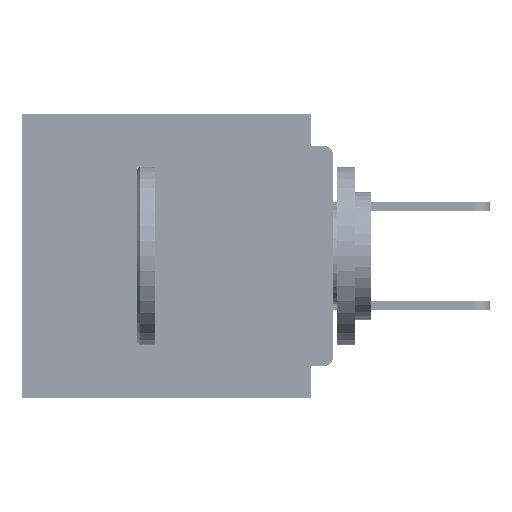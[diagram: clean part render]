
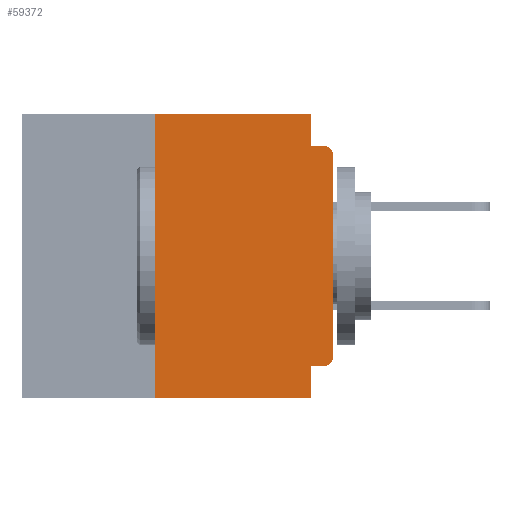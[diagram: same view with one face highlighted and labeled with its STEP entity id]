
A CAD part, left-side view. The second image highlights one B-rep face of the part: STEP entity #59372.
In plain terms, the highlighted planar face has unit normal (-1, 0, 0).
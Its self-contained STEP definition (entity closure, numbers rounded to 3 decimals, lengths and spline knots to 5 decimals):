
#410 = ORIENTED_EDGE ( 'NONE', *, *, #3255, .T. ) ;
#1782 = CARTESIAN_POINT ( 'NONE',  ( 0., 0.437, 0. ) ) ;
#1828 = CARTESIAN_POINT ( 'NONE',  ( 0., 0.437, -0.4 ) ) ;
#3255 = EDGE_CURVE ( 'NONE', #49868, #56918, #58562, .T. ) ;
#4190 = EDGE_CURVE ( 'NONE', #19603, #50509, #42094, .T. ) ;
#5591 = LINE ( 'NONE', #66463, #33182 ) ;
#6256 = DIRECTION ( 'NONE',  ( 0., 0., -1. ) ) ;
#6961 = CARTESIAN_POINT ( 'NONE',  ( 0., 0., -0.06 ) ) ;
#8566 = CARTESIAN_POINT ( 'NONE',  ( 0., 0.031, -0.045 ) ) ;
#9851 = CIRCLE ( 'NONE', #39563, 0.015 ) ;
#10438 = DIRECTION ( 'NONE',  ( 0., 0., 1. ) ) ;
#12716 = VECTOR ( 'NONE', #30200, 39.37008 ) ;
#12919 = DIRECTION ( 'NONE',  ( 0., -1., 0. ) ) ;
#14512 = ORIENTED_EDGE ( 'NONE', *, *, #43655, .F. ) ;
#14680 = VECTOR ( 'NONE', #12919, 39.37008 ) ;
#15242 = LINE ( 'NONE', #63293, #57412 ) ;
#17301 = DIRECTION ( 'NONE',  ( 0., 0., 1. ) ) ;
#17589 = ORIENTED_EDGE ( 'NONE', *, *, #36982, .F. ) ;
#17661 = VECTOR ( 'NONE', #10438, 39.37008 ) ;
#17810 = ORIENTED_EDGE ( 'NONE', *, *, #57782, .T. ) ;
#17824 = LINE ( 'NONE', #28598, #30752 ) ;
#18502 = CARTESIAN_POINT ( 'NONE',  ( 0., 0.015, -0.355 ) ) ;
#19491 = DIRECTION ( 'NONE',  ( 0., -1., 0. ) ) ;
#19603 = VERTEX_POINT ( 'NONE', #49033 ) ;
#23544 = VERTEX_POINT ( 'NONE', #53083 ) ;
#24085 = VERTEX_POINT ( 'NONE', #58064 ) ;
#24659 = CARTESIAN_POINT ( 'NONE',  ( 0., 0.031, -0.4 ) ) ;
#24747 = CIRCLE ( 'NONE', #70705, 0.015 ) ;
#24909 = CARTESIAN_POINT ( 'NONE',  ( 0., 0.031, -0.355 ) ) ;
#25709 = VECTOR ( 'NONE', #71172, 39.37008 ) ;
#27699 = EDGE_CURVE ( 'NONE', #38769, #59005, #9851, .T. ) ;
#27729 = DIRECTION ( 'NONE',  ( -1., 0., 0. ) ) ;
#28598 = CARTESIAN_POINT ( 'NONE',  ( 0., 0.25, -0.4 ) ) ;
#29008 = EDGE_LOOP ( 'NONE', ( #17810, #35848, #32737, #31289, #31049, #14512, #410, #48712, #17589, #31955 ) ) ;
#29044 = CARTESIAN_POINT ( 'NONE',  ( 0., 0.015, -0.06 ) ) ;
#30200 = DIRECTION ( 'NONE',  ( 0., 0., -1. ) ) ;
#30752 = VECTOR ( 'NONE', #17301, 39.37008 ) ;
#31049 = ORIENTED_EDGE ( 'NONE', *, *, #34780, .F. ) ;
#31289 = ORIENTED_EDGE ( 'NONE', *, *, #4190, .F. ) ;
#31955 = ORIENTED_EDGE ( 'NONE', *, *, #34405, .T. ) ;
#32536 = LINE ( 'NONE', #24659, #12716 ) ;
#32737 = ORIENTED_EDGE ( 'NONE', *, *, #57930, .F. ) ;
#33182 = VECTOR ( 'NONE', #39047, 39.37008 ) ;
#33300 = VECTOR ( 'NONE', #45687, 39.37008 ) ;
#34405 = EDGE_CURVE ( 'NONE', #64531, #23544, #24747, .T. ) ;
#34609 = DIRECTION ( 'NONE',  ( 0., 0., -1. ) ) ;
#34780 = EDGE_CURVE ( 'NONE', #24085, #19603, #15242, .T. ) ;
#35848 = ORIENTED_EDGE ( 'NONE', *, *, #27699, .T. ) ;
#36982 = EDGE_CURVE ( 'NONE', #64531, #40003, #62532, .T. ) ;
#38769 = VERTEX_POINT ( 'NONE', #6961 ) ;
#38946 = FACE_OUTER_BOUND ( 'NONE', #29008, .T. ) ;
#39047 = DIRECTION ( 'NONE',  ( 0., -1., 0. ) ) ;
#39563 = AXIS2_PLACEMENT_3D ( 'NONE', #29044, #67513, #34609 ) ;
#40003 = VERTEX_POINT ( 'NONE', #24909 ) ;
#40141 = CARTESIAN_POINT ( 'NONE',  ( 0., 0., -0.355 ) ) ;
#40300 = PLANE ( 'NONE',  #56675 ) ;
#42094 = LINE ( 'NONE', #65665, #25709 ) ;
#42560 = EDGE_CURVE ( 'NONE', #40003, #56918, #32536, .T. ) ;
#43394 = CARTESIAN_POINT ( 'NONE',  ( 0., 0., 0. ) ) ;
#43655 = EDGE_CURVE ( 'NONE', #49868, #24085, #17824, .T. ) ;
#45687 = DIRECTION ( 'NONE',  ( 0., 1., 0. ) ) ;
#48712 = ORIENTED_EDGE ( 'NONE', *, *, #42560, .F. ) ;
#49033 = CARTESIAN_POINT ( 'NONE',  ( 0., 0.031, 0. ) ) ;
#49868 = VERTEX_POINT ( 'NONE', #69228 ) ;
#50509 = VERTEX_POINT ( 'NONE', #8566 ) ;
#53083 = CARTESIAN_POINT ( 'NONE',  ( 0., 0., -0.34 ) ) ;
#56675 = AXIS2_PLACEMENT_3D ( 'NONE', #1782, #65599, #6256 ) ;
#56918 = VERTEX_POINT ( 'NONE', #62493 ) ;
#57412 = VECTOR ( 'NONE', #19491, 39.37008 ) ;
#57782 = EDGE_CURVE ( 'NONE', #23544, #38769, #58117, .T. ) ;
#57930 = EDGE_CURVE ( 'NONE', #50509, #59005, #5591, .T. ) ;
#58064 = CARTESIAN_POINT ( 'NONE',  ( 0., 0.25, 0. ) ) ;
#58117 = LINE ( 'NONE', #43394, #17661 ) ;
#58562 = LINE ( 'NONE', #1828, #14680 ) ;
#59005 = VERTEX_POINT ( 'NONE', #64841 ) ;
#59372 = ADVANCED_FACE ( 'NONE', ( #38946 ), #40300, .F. ) ;
#60688 = CARTESIAN_POINT ( 'NONE',  ( 0., 0.015, -0.34 ) ) ;
#62493 = CARTESIAN_POINT ( 'NONE',  ( 0., 0.031, -0.4 ) ) ;
#62532 = LINE ( 'NONE', #40141, #33300 ) ;
#63293 = CARTESIAN_POINT ( 'NONE',  ( 0., 0.437, 0. ) ) ;
#64531 = VERTEX_POINT ( 'NONE', #18502 ) ;
#64841 = CARTESIAN_POINT ( 'NONE',  ( 0., 0.015, -0.045 ) ) ;
#65599 = DIRECTION ( 'NONE',  ( 1., 0., 0. ) ) ;
#65665 = CARTESIAN_POINT ( 'NONE',  ( 0., 0.031, 0. ) ) ;
#66218 = DIRECTION ( 'NONE',  ( 0., 0., -1. ) ) ;
#66463 = CARTESIAN_POINT ( 'NONE',  ( 0., 0., -0.045 ) ) ;
#67513 = DIRECTION ( 'NONE',  ( -1., 0., 0. ) ) ;
#69228 = CARTESIAN_POINT ( 'NONE',  ( 0., 0.25, -0.4 ) ) ;
#70705 = AXIS2_PLACEMENT_3D ( 'NONE', #60688, #27729, #66218 ) ;
#71172 = DIRECTION ( 'NONE',  ( 0., 0., -1. ) ) ;
